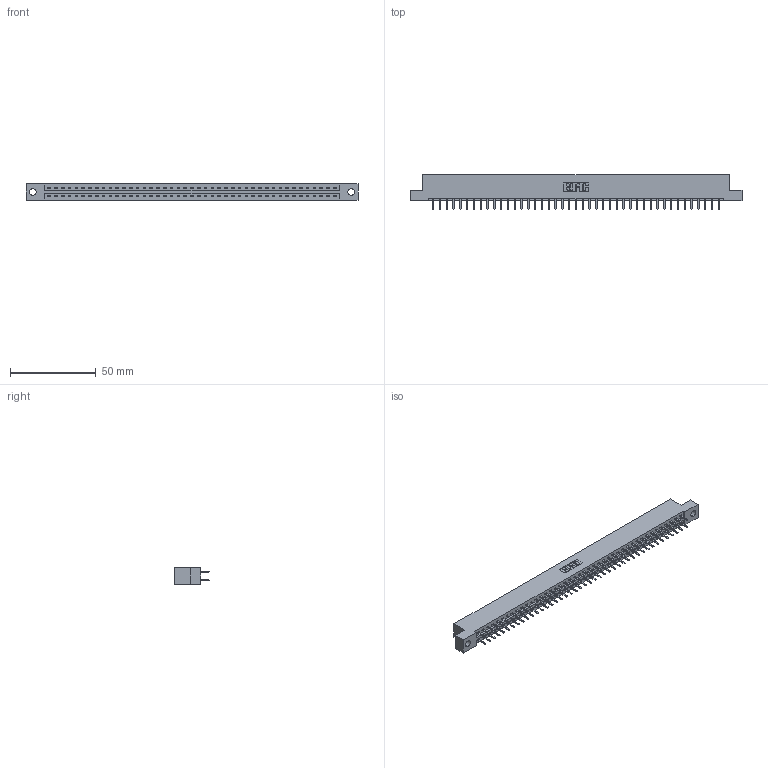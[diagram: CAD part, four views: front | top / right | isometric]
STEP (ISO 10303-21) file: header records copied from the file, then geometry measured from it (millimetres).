
FILE_DESCRIPTION (( 'STEP AP203' ), '1' );
FILE_NAME ('387-086-520-204.STEP', '2018-09-23T23:12:09', ( '' ), ( '' ), 'SwSTEP 2.0', 'SolidWorks 2016', '' );
FILE_SCHEMA (( 'CONFIG_CONTROL_DESIGN' ));
Length unit declared in the file: inch
Products named in the file (3): 337 Part_Flush Mounting Lugs - 0.156 Dia-TH; 345-292-001_345-293-120; 387-086-520-204
Assembly tree (87 placements, depth 2):
  387-086-520-204
    337 Part_Flush Mounting Lugs - 0.156 Dia-TH
    345-292-001_345-293-120  x86
Bounding box: 193.4 x 20.02 x 9.4 mm (x, y, z)
Volume: 20269.2 mm3; surface area: 22613.7 mm2
Topology: 87 solids, 87 shells, 5102 faces, 14845 edges, 9666 vertices
Faces by surface type: plane 3510, cylinder 1592
Entity records: 33327 total; most frequent: CARTESIAN_POINT 5626, ORIENTED_EDGE 5550, DIRECTION 4771, EDGE_CURVE 2775, LINE 2643, VECTOR 2643, VERTEX_POINT 1846, AXIS2_PLACEMENT_3D 1064
